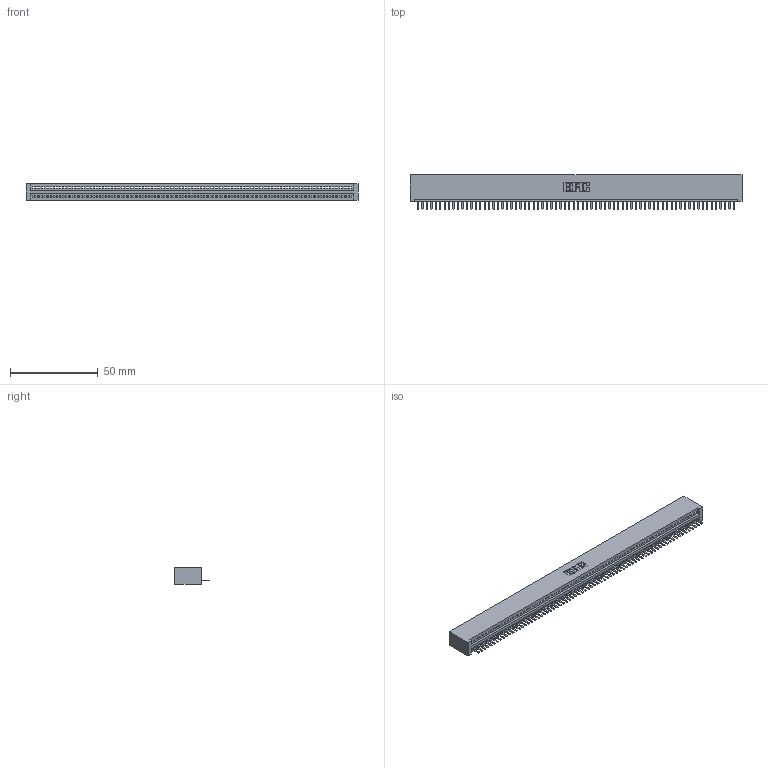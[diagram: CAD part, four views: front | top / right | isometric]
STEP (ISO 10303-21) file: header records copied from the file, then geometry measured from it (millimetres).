
FILE_DESCRIPTION (( 'STEP AP203' ), '1' );
FILE_NAME ('345-072-520-101.STEP', '2018-10-01T18:00:48', ( '' ), ( '' ), 'SwSTEP 2.0', 'SolidWorks 2016', '' );
FILE_SCHEMA (( 'CONFIG_CONTROL_DESIGN' ));
Length unit declared in the file: inch
Products named in the file (3): 345 Part_No Mounting Lugs; 345-072-520-101; 345-292-001_345-293-120
Assembly tree (73 placements, depth 2):
  345-072-520-101
    345 Part_No Mounting Lugs
    345-292-001_345-293-120  x72
Bounding box: 189.48 x 19.68 x 9.4 mm (x, y, z)
Volume: 18620.4 mm3; surface area: 24665.1 mm2
Topology: 73 solids, 73 shells, 4582 faces, 13565 edges, 8850 vertices
Faces by surface type: plane 3100, cylinder 1482
Entity records: 49987 total; most frequent: CARTESIAN_POINT 8676, ORIENTED_EDGE 8670, DIRECTION 7515, EDGE_CURVE 4335, LINE 3919, VECTOR 3919, VERTEX_POINT 2886, AXIS2_PLACEMENT_3D 1798
